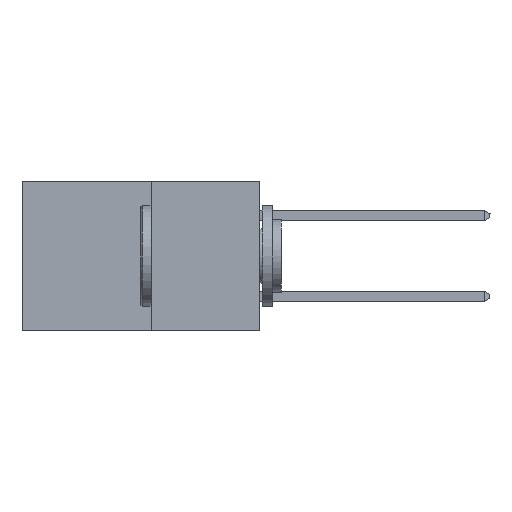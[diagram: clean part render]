
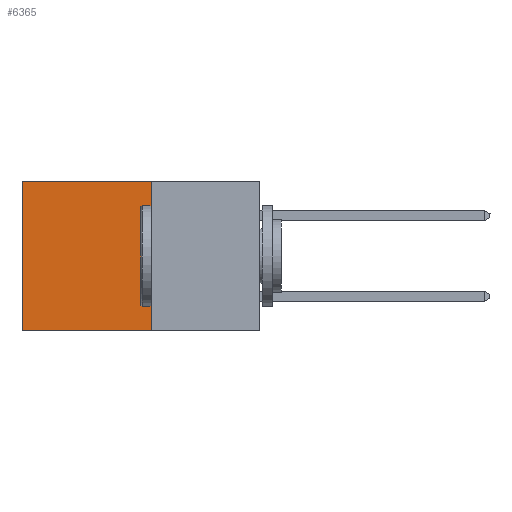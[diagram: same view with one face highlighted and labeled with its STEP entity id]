
A CAD part, left-side view. The second image highlights one B-rep face of the part: STEP entity #6365.
In plain terms, the highlighted planar face has unit normal (-1, 0, 0).
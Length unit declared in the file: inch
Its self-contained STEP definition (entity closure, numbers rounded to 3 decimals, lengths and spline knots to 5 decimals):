
#1039 = DIRECTION ( 'NONE',  ( 0., 1., 0. ) ) ;
#1097 = CARTESIAN_POINT ( 'NONE',  ( 0.277, 0.59, -0.37 ) ) ;
#1254 = LINE ( 'NONE', #9411, #4275 ) ;
#1702 = VECTOR ( 'NONE', #3411, 39.37008 ) ;
#1861 = CARTESIAN_POINT ( 'NONE',  ( 0.277, 0.27, -0.37 ) ) ;
#2290 = VERTEX_POINT ( 'NONE', #1861 ) ;
#2585 = LINE ( 'NONE', #11781, #13562 ) ;
#2615 = LINE ( 'NONE', #14179, #7806 ) ;
#3210 = DIRECTION ( 'NONE',  ( 0., 0., -1. ) ) ;
#3411 = DIRECTION ( 'NONE',  ( 0., 0., -1. ) ) ;
#4275 = VECTOR ( 'NONE', #10513, 39.37008 ) ;
#4411 = EDGE_LOOP ( 'NONE', ( #5141, #6707, #6824, #6901 ) ) ;
#4566 = AXIS2_PLACEMENT_3D ( 'NONE', #14097, #9787, #3210 ) ;
#5141 = ORIENTED_EDGE ( 'NONE', *, *, #6481, .T. ) ;
#6365 = ADVANCED_FACE ( 'NONE', ( #12528 ), #13008, .F. ) ;
#6481 = EDGE_CURVE ( 'NONE', #7328, #10595, #7588, .T. ) ;
#6707 = ORIENTED_EDGE ( 'NONE', *, *, #11330, .F. ) ;
#6824 = ORIENTED_EDGE ( 'NONE', *, *, #8307, .F. ) ;
#6901 = ORIENTED_EDGE ( 'NONE', *, *, #13083, .T. ) ;
#7128 = CARTESIAN_POINT ( 'NONE',  ( 0.277, 0.59, -0.37 ) ) ;
#7328 = VERTEX_POINT ( 'NONE', #9142 ) ;
#7588 = LINE ( 'NONE', #1097, #1702 ) ;
#7806 = VECTOR ( 'NONE', #1039, 39.37008 ) ;
#8307 = EDGE_CURVE ( 'NONE', #9139, #2290, #2585, .T. ) ;
#9139 = VERTEX_POINT ( 'NONE', #10043 ) ;
#9142 = CARTESIAN_POINT ( 'NONE',  ( 0.277, 0.59, 0. ) ) ;
#9411 = CARTESIAN_POINT ( 'NONE',  ( 0.277, 0.27, -0.37 ) ) ;
#9787 = DIRECTION ( 'NONE',  ( 1., 0., 0. ) ) ;
#10043 = CARTESIAN_POINT ( 'NONE',  ( 0.277, 0.27, 0. ) ) ;
#10513 = DIRECTION ( 'NONE',  ( 0., 1., 0. ) ) ;
#10595 = VERTEX_POINT ( 'NONE', #7128 ) ;
#11330 = EDGE_CURVE ( 'NONE', #2290, #10595, #1254, .T. ) ;
#11781 = CARTESIAN_POINT ( 'NONE',  ( 0.277, 0.27, -0.37 ) ) ;
#12528 = FACE_OUTER_BOUND ( 'NONE', #4411, .T. ) ;
#13008 = PLANE ( 'NONE',  #4566 ) ;
#13083 = EDGE_CURVE ( 'NONE', #9139, #7328, #2615, .T. ) ;
#13562 = VECTOR ( 'NONE', #13954, 39.37008 ) ;
#13954 = DIRECTION ( 'NONE',  ( 0., 0., -1. ) ) ;
#14097 = CARTESIAN_POINT ( 'NONE',  ( 0.277, 0.27, -0.37 ) ) ;
#14179 = CARTESIAN_POINT ( 'NONE',  ( 0.277, 0.27, 0. ) ) ;
